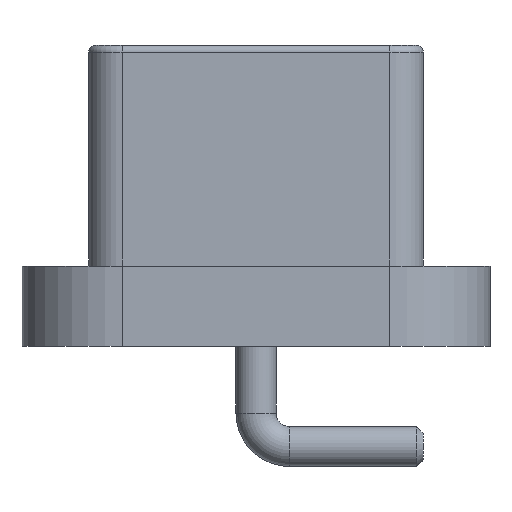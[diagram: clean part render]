
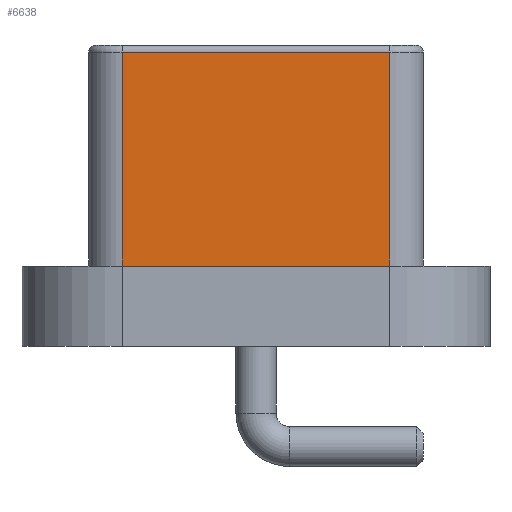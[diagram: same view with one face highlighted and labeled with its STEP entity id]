
A CAD part, left-side view. The second image highlights one B-rep face of the part: STEP entity #6638.
In plain terms, the highlighted planar face has unit normal (-1, 0, 0).
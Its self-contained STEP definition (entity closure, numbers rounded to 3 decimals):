
#1176 = DIRECTION ( 'NONE',  ( 1., 0., 0. ) ) ;
#1344 = CARTESIAN_POINT ( 'NONE',  ( -9.65, -2., -0.1 ) ) ;
#2466 = LINE ( 'NONE', #4325, #4071 ) ;
#2629 = DIRECTION ( 'NONE',  ( 0., -1., 0. ) ) ;
#2732 = VERTEX_POINT ( 'NONE', #11681 ) ;
#2912 = CARTESIAN_POINT ( 'NONE',  ( -9.65, -2., -3.3 ) ) ;
#2939 = ORIENTED_EDGE ( 'NONE', *, *, #3166, .T. ) ;
#3166 = EDGE_CURVE ( 'NONE', #2732, #4631, #8297, .T. ) ;
#3880 = VECTOR ( 'NONE', #6495, 1000. ) ;
#4071 = VECTOR ( 'NONE', #7982, 1000. ) ;
#4325 = CARTESIAN_POINT ( 'NONE',  ( -9.65, 2., -0.1 ) ) ;
#4631 = VERTEX_POINT ( 'NONE', #9624 ) ;
#4911 = VECTOR ( 'NONE', #5970, 1000. ) ;
#5341 = EDGE_CURVE ( 'NONE', #4631, #9977, #8871, .T. ) ;
#5627 = ORIENTED_EDGE ( 'NONE', *, *, #5341, .T. ) ;
#5628 = CARTESIAN_POINT ( 'NONE',  ( -9.65, 2., -0.1 ) ) ;
#5684 = DIRECTION ( 'NONE',  ( 0., 1., 0. ) ) ;
#5743 = FACE_OUTER_BOUND ( 'NONE', #10295, .T. ) ;
#5970 = DIRECTION ( 'NONE',  ( 0., 1., 0. ) ) ;
#6072 = ORIENTED_EDGE ( 'NONE', *, *, #10239, .T. ) ;
#6215 = CARTESIAN_POINT ( 'NONE',  ( -9.65, 2., -3.3 ) ) ;
#6229 = CARTESIAN_POINT ( 'NONE',  ( -9.65, 2., -3.3 ) ) ;
#6495 = DIRECTION ( 'NONE',  ( 0., 0., 1. ) ) ;
#6638 = ADVANCED_FACE ( 'NONE', ( #5743 ), #6701, .F. ) ;
#6701 = PLANE ( 'NONE',  #7429 ) ;
#6767 = CARTESIAN_POINT ( 'NONE',  ( -9.65, 0., -1.7 ) ) ;
#6939 = VECTOR ( 'NONE', #2629, 1000. ) ;
#7429 = AXIS2_PLACEMENT_3D ( 'NONE', #6767, #1176, #5684 ) ;
#7982 = DIRECTION ( 'NONE',  ( 0., 0., -1. ) ) ;
#8192 = ORIENTED_EDGE ( 'NONE', *, *, #9910, .T. ) ;
#8297 = LINE ( 'NONE', #2912, #3880 ) ;
#8871 = LINE ( 'NONE', #1344, #4911 ) ;
#9151 = VERTEX_POINT ( 'NONE', #6215 ) ;
#9624 = CARTESIAN_POINT ( 'NONE',  ( -9.65, -2., -0.1 ) ) ;
#9910 = EDGE_CURVE ( 'NONE', #9151, #2732, #9962, .T. ) ;
#9962 = LINE ( 'NONE', #6229, #6939 ) ;
#9977 = VERTEX_POINT ( 'NONE', #5628 ) ;
#10239 = EDGE_CURVE ( 'NONE', #9977, #9151, #2466, .T. ) ;
#10295 = EDGE_LOOP ( 'NONE', ( #6072, #8192, #2939, #5627 ) ) ;
#11681 = CARTESIAN_POINT ( 'NONE',  ( -9.65, -2., -3.3 ) ) ;
